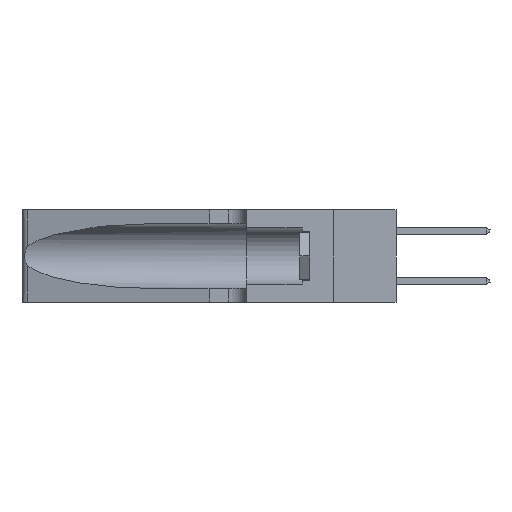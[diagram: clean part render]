
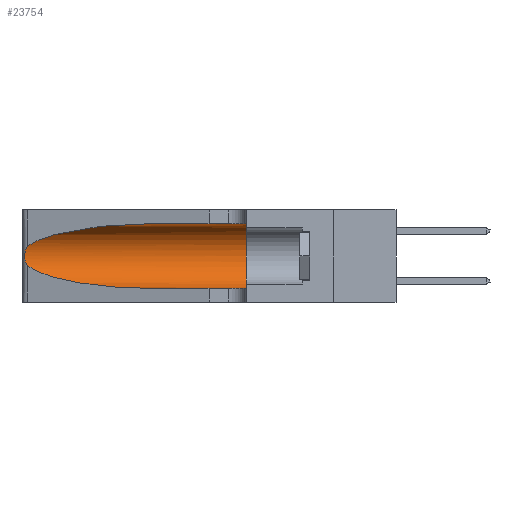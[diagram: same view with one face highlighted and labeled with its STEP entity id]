
A CAD part, left-side view. The second image highlights one B-rep face of the part: STEP entity #23754.
In plain terms, the highlighted cylindrical face has radius 3.308 mm (diameter 6.617 mm), a partial arc.
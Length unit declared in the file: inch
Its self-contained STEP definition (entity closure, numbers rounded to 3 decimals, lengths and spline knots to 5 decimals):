
#395 = DIRECTION ( 'NONE',  ( 0., -1., 0. ) ) ;
#1312 = DIRECTION ( 'NONE',  ( 0., 0., -1. ) ) ;
#1684 =( BOUNDED_CURVE ( )  B_SPLINE_CURVE ( 3, ( #29456, #14296, #20453, #1965 ),
 .UNSPECIFIED., .F., .F. ) 
 B_SPLINE_CURVE_WITH_KNOTS ( ( 4, 4 ),
 ( 3.44316, 4.71239 ),
 .UNSPECIFIED. ) 
 CURVE ( )  GEOMETRIC_REPRESENTATION_ITEM ( )  RATIONAL_B_SPLINE_CURVE ( ( 1., 0.87, 0.87, 1. ) ) 
 REPRESENTATION_ITEM ( '' )  );
#1965 = CARTESIAN_POINT ( 'NONE',  ( 0.1305, 0.72297, 0.05475 ) ) ;
#3067 = CARTESIAN_POINT ( 'NONE',  ( 0.25555, 1.22993, 0.14849 ) ) ;
#3908 = ORIENTED_EDGE ( 'NONE', *, *, #34067, .T. ) ;
#4509 = DIRECTION ( 'NONE',  ( 0., -1., 0. ) ) ;
#4676 = VERTEX_POINT ( 'NONE', #35862 ) ;
#4775 = EDGE_CURVE ( 'NONE', #16125, #29556, #37085, .T. ) ;
#5043 = DIRECTION ( 'NONE',  ( 0., -1., 0. ) ) ;
#5848 = CARTESIAN_POINT ( 'NONE',  ( 0.1305, 0.72297, 0.31525 ) ) ;
#6504 = FACE_OUTER_BOUND ( 'NONE', #23268, .T. ) ;
#6559 = AXIS2_PLACEMENT_3D ( 'NONE', #13237, #34492, #16338 ) ;
#6737 = ORIENTED_EDGE ( 'NONE', *, *, #4775, .T. ) ;
#7648 = CARTESIAN_POINT ( 'NONE',  ( 0.1305, 1.61858, 0.185 ) ) ;
#9183 = CARTESIAN_POINT ( 'NONE',  ( 0.25787, 1.23484, 0.2124 ) ) ;
#9817 = AXIS2_PLACEMENT_3D ( 'NONE', #7648, #4509, #1312 ) ;
#10749 = CIRCLE ( 'NONE', #6559, 0.13025 ) ;
#11493 = ORIENTED_EDGE ( 'NONE', *, *, #23279, .T. ) ;
#12126 = ORIENTED_EDGE ( 'NONE', *, *, #17258, .F. ) ;
#12301 = CARTESIAN_POINT ( 'NONE',  ( 0.26018, 1.23835, 0.19895 ) ) ;
#12758 = CARTESIAN_POINT ( 'NONE',  ( 0.1305, 0.72297, 0.31525 ) ) ;
#13237 = CARTESIAN_POINT ( 'NONE',  ( 0.1305, 0.35, 0.185 ) ) ;
#13769 = VECTOR ( 'NONE', #5043, 39.37008 ) ;
#14296 = CARTESIAN_POINT ( 'NONE',  ( 0.2373, 1.15595, 0.08982 ) ) ;
#15387 = CARTESIAN_POINT ( 'NONE',  ( 0.26075, 1.23896, 0.178 ) ) ;
#15973 = ORIENTED_EDGE ( 'NONE', *, *, #17154, .T. ) ;
#16125 = VERTEX_POINT ( 'NONE', #12758 ) ;
#16338 = DIRECTION ( 'NONE',  ( 0., 0., 1. ) ) ;
#17154 = EDGE_CURVE ( 'NONE', #29556, #27004, #35618, .T. ) ;
#17258 = EDGE_CURVE ( 'NONE', #16125, #4676, #26058, .T. ) ;
#17717 = EDGE_CURVE ( 'NONE', #4676, #25685, #10749, .T. ) ;
#18030 = VECTOR ( 'NONE', #395, 39.37008 ) ;
#18473 = CARTESIAN_POINT ( 'NONE',  ( 0.25856, 1.23593, 0.16098 ) ) ;
#19952 = CYLINDRICAL_SURFACE ( 'NONE', #9817, 0.13025 ) ;
#20453 = CARTESIAN_POINT ( 'NONE',  ( 0.18966, 0.96281, 0.05475 ) ) ;
#21376 = CARTESIAN_POINT ( 'NONE',  ( 0.25555, 1.22994, 0.2215 ) ) ;
#21489 = CARTESIAN_POINT ( 'NONE',  ( 0.25639, 1.23186, 0.15144 ) ) ;
#21874 = LINE ( 'NONE', #38512, #13769 ) ;
#22750 = CARTESIAN_POINT ( 'NONE',  ( 0.1305, 0.35, 0.05475 ) ) ;
#23268 = EDGE_LOOP ( 'NONE', ( #6737, #15973, #3908, #11493, #27523, #12126 ) ) ;
#23279 = EDGE_CURVE ( 'NONE', #23513, #25685, #21874, .T. ) ;
#23365 = CARTESIAN_POINT ( 'NONE',  ( 0.25487, 1.22718, 0.22369 ) ) ;
#23513 = VERTEX_POINT ( 'NONE', #37174 ) ;
#23754 = ADVANCED_FACE ( 'NONE', ( #6504 ), #19952, .F. ) ;
#24194 = CARTESIAN_POINT ( 'NONE',  ( 0.18966, 0.96281, 0.31525 ) ) ;
#24426 = CARTESIAN_POINT ( 'NONE',  ( 0.25487, 1.22718, 0.22369 ) ) ;
#24539 = CARTESIAN_POINT ( 'NONE',  ( 0.25487, 1.22718, 0.14631 ) ) ;
#25685 = VERTEX_POINT ( 'NONE', #22750 ) ;
#26058 = LINE ( 'NONE', #31031, #18030 ) ;
#27004 = VERTEX_POINT ( 'NONE', #35094 ) ;
#27111 = CARTESIAN_POINT ( 'NONE',  ( 0.2373, 1.15595, 0.28018 ) ) ;
#27240 = CARTESIAN_POINT ( 'NONE',  ( 0.25487, 1.22718, 0.22369 ) ) ;
#27462 = CARTESIAN_POINT ( 'NONE',  ( 0.25639, 1.23184, 0.21858 ) ) ;
#27523 = ORIENTED_EDGE ( 'NONE', *, *, #17717, .F. ) ;
#29456 = CARTESIAN_POINT ( 'NONE',  ( 0.25487, 1.22718, 0.14631 ) ) ;
#29556 = VERTEX_POINT ( 'NONE', #23365 ) ;
#30506 = CARTESIAN_POINT ( 'NONE',  ( 0.25854, 1.2359, 0.20912 ) ) ;
#31031 = CARTESIAN_POINT ( 'NONE',  ( 0.1305, 1.61858, 0.31525 ) ) ;
#33565 = CARTESIAN_POINT ( 'NONE',  ( 0.26075, 1.23896, 0.19203 ) ) ;
#34067 = EDGE_CURVE ( 'NONE', #27004, #23513, #1684, .T. ) ;
#34492 = DIRECTION ( 'NONE',  ( 0., 1., 0. ) ) ;
#35094 = CARTESIAN_POINT ( 'NONE',  ( 0.25487, 1.22718, 0.14631 ) ) ;
#35618 = B_SPLINE_CURVE_WITH_KNOTS ( 'NONE', 3,
 ( #24426, #21376, #27462, #9183, #30506, #12301, #33565, #15387, #36607, #18473, #39651, #21489, #3067, #24539 ),
 .UNSPECIFIED., .F., .F.,
 ( 4, 2, 2, 2, 2, 2, 4 ),
 ( 0., 0.00027, 0.00053, 0.00107, 0.0016, 0.00187, 0.00214 ),
 .UNSPECIFIED. ) ;
#35862 = CARTESIAN_POINT ( 'NONE',  ( 0.1305, 0.35, 0.31525 ) ) ;
#36607 = CARTESIAN_POINT ( 'NONE',  ( 0.26017, 1.23833, 0.17102 ) ) ;
#37085 =( BOUNDED_CURVE ( )  B_SPLINE_CURVE ( 3, ( #5848, #24194, #27111, #27240 ),
 .UNSPECIFIED., .F., .T. ) 
 B_SPLINE_CURVE_WITH_KNOTS ( ( 4, 4 ),
 ( 1.5708, 2.84003 ),
 .UNSPECIFIED. ) 
 CURVE ( )  GEOMETRIC_REPRESENTATION_ITEM ( )  RATIONAL_B_SPLINE_CURVE ( ( 1., 0.87, 0.87, 1. ) ) 
 REPRESENTATION_ITEM ( '' )  );
#37174 = CARTESIAN_POINT ( 'NONE',  ( 0.1305, 0.72297, 0.05475 ) ) ;
#38512 = CARTESIAN_POINT ( 'NONE',  ( 0.1305, 1.61858, 0.05475 ) ) ;
#39651 = CARTESIAN_POINT ( 'NONE',  ( 0.25789, 1.23486, 0.15765 ) ) ;
